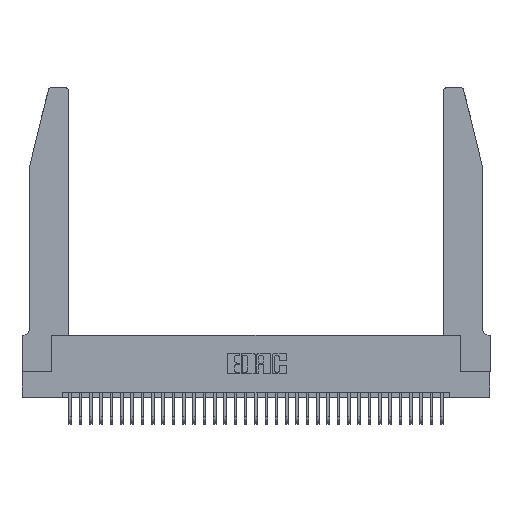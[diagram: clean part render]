
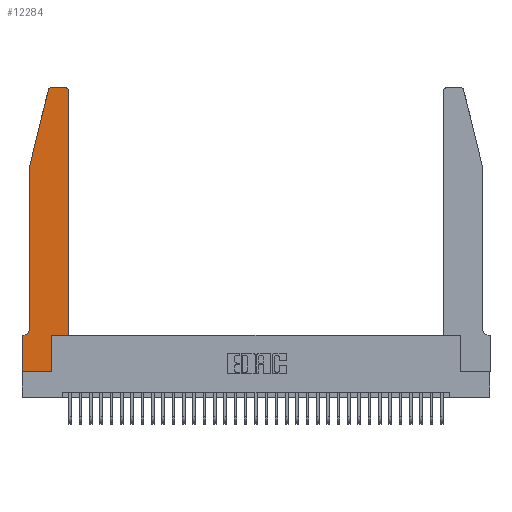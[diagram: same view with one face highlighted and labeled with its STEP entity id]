
A CAD part, top view. The second image highlights one B-rep face of the part: STEP entity #12284.
In plain terms, the highlighted planar face has unit normal (0, 0, 1).
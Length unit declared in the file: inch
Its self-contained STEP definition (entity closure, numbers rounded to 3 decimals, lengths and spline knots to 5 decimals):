
#522 = EDGE_CURVE ( 'NONE', #15158, #9549, #29890, .T. ) ;
#568 = LINE ( 'NONE', #18574, #27272 ) ;
#1459 = DIRECTION ( 'NONE',  ( -1., 0., 0. ) ) ;
#1544 = DIRECTION ( 'NONE',  ( 0., 0., 1. ) ) ;
#1998 = FACE_OUTER_BOUND ( 'NONE', #5736, .T. ) ;
#2839 = CARTESIAN_POINT ( 'NONE',  ( 0.0755, 2., 0.37 ) ) ;
#2873 = CARTESIAN_POINT ( 'NONE',  ( 0.2865, 0., 0.37 ) ) ;
#3316 = CARTESIAN_POINT ( 'NONE',  ( 0.4205, 2.75, 0.37 ) ) ;
#3374 = EDGE_CURVE ( 'NONE', #4253, #15158, #20533, .T. ) ;
#4253 = VERTEX_POINT ( 'NONE', #31362 ) ;
#4255 = EDGE_CURVE ( 'NONE', #18938, #19141, #568, .T. ) ;
#4879 = VERTEX_POINT ( 'NONE', #28804 ) ;
#4895 = DIRECTION ( 'NONE',  ( 0., 0., 1. ) ) ;
#5441 = CARTESIAN_POINT ( 'NONE',  ( 0.4505, 0.35, 0.37 ) ) ;
#5593 = EDGE_CURVE ( 'NONE', #32367, #4879, #26120, .T. ) ;
#5736 = EDGE_LOOP ( 'NONE', ( #17999, #22004, #30364, #19204, #9488, #18029, #5848, #23654, #18455, #13189, #17225, #11971 ) ) ;
#5848 = ORIENTED_EDGE ( 'NONE', *, *, #13122, .T. ) ;
#5872 = DIRECTION ( 'NONE',  ( 0., 0., -1. ) ) ;
#7199 = CARTESIAN_POINT ( 'NONE',  ( 0.0755, 0.42, 0.37 ) ) ;
#7503 = EDGE_CURVE ( 'NONE', #4879, #18938, #32324, .T. ) ;
#7509 = AXIS2_PLACEMENT_3D ( 'NONE', #8967, #26994, #11577 ) ;
#8612 = VECTOR ( 'NONE', #14992, 39.37008 ) ;
#8967 = CARTESIAN_POINT ( 'NONE',  ( 0.284, 2.72, 0.37 ) ) ;
#9488 = ORIENTED_EDGE ( 'NONE', *, *, #32392, .T. ) ;
#9549 = VERTEX_POINT ( 'NONE', #17577 ) ;
#9755 = CARTESIAN_POINT ( 'NONE',  ( 0., 0., 0.37 ) ) ;
#10136 = EDGE_CURVE ( 'NONE', #9549, #29357, #19407, .T. ) ;
#10212 = CARTESIAN_POINT ( 'NONE',  ( 0.2605, 2.75, 0.37 ) ) ;
#10248 = LINE ( 'NONE', #17865, #22350 ) ;
#11153 = LINE ( 'NONE', #19621, #17193 ) ;
#11577 = DIRECTION ( 'NONE',  ( 1., 0., 0. ) ) ;
#11908 = VECTOR ( 'NONE', #29328, 39.37008 ) ;
#11971 = ORIENTED_EDGE ( 'NONE', *, *, #10136, .T. ) ;
#12284 = ADVANCED_FACE ( 'NONE', ( #1998 ), #32400, .T. ) ;
#13122 = EDGE_CURVE ( 'NONE', #14083, #20221, #17404, .T. ) ;
#13189 = ORIENTED_EDGE ( 'NONE', *, *, #3374, .T. ) ;
#13206 = EDGE_CURVE ( 'NONE', #29357, #32367, #13377, .T. ) ;
#13377 = LINE ( 'NONE', #10212, #26264 ) ;
#14083 = VERTEX_POINT ( 'NONE', #29036 ) ;
#14992 = DIRECTION ( 'NONE',  ( 1., 0., 0. ) ) ;
#15158 = VERTEX_POINT ( 'NONE', #27956 ) ;
#15182 = DIRECTION ( 'NONE',  ( 0., 1., 0. ) ) ;
#15446 = DIRECTION ( 'NONE',  ( -1., 0., 0. ) ) ;
#15706 = VERTEX_POINT ( 'NONE', #23068 ) ;
#17193 = VECTOR ( 'NONE', #1459, 39.37008 ) ;
#17225 = ORIENTED_EDGE ( 'NONE', *, *, #522, .T. ) ;
#17404 = LINE ( 'NONE', #32818, #23449 ) ;
#17577 = CARTESIAN_POINT ( 'NONE',  ( 0.4505, 2.72, 0.37 ) ) ;
#17865 = CARTESIAN_POINT ( 'NONE',  ( 0.2865, 0.35, 0.37 ) ) ;
#17999 = ORIENTED_EDGE ( 'NONE', *, *, #13206, .T. ) ;
#18029 = ORIENTED_EDGE ( 'NONE', *, *, #19073, .T. ) ;
#18455 = ORIENTED_EDGE ( 'NONE', *, *, #32812, .T. ) ;
#18574 = CARTESIAN_POINT ( 'NONE',  ( 0.0755, 2., 0.37 ) ) ;
#18680 = DIRECTION ( 'NONE',  ( 0., -1., 0. ) ) ;
#18938 = VERTEX_POINT ( 'NONE', #2839 ) ;
#19073 = EDGE_CURVE ( 'NONE', #15706, #14083, #11153, .T. ) ;
#19141 = VERTEX_POINT ( 'NONE', #7199 ) ;
#19204 = ORIENTED_EDGE ( 'NONE', *, *, #4255, .T. ) ;
#19407 = CIRCLE ( 'NONE', #25103, 0.03 ) ;
#19621 = CARTESIAN_POINT ( 'NONE',  ( 0.0755, 0.35, 0.37 ) ) ;
#19713 = DIRECTION ( 'NONE',  ( 1., 0., 0. ) ) ;
#20221 = VERTEX_POINT ( 'NONE', #29180 ) ;
#20427 = CARTESIAN_POINT ( 'NONE',  ( 0.4205, 2.72, 0.37 ) ) ;
#20432 = DIRECTION ( 'NONE',  ( 0., 1., 0. ) ) ;
#20533 = LINE ( 'NONE', #5441, #32455 ) ;
#21373 = CARTESIAN_POINT ( 'NONE',  ( 0.0055, 0.42, 0.37 ) ) ;
#22004 = ORIENTED_EDGE ( 'NONE', *, *, #5593, .T. ) ;
#22350 = VECTOR ( 'NONE', #20432, 39.37008 ) ;
#22750 = DIRECTION ( 'NONE',  ( 0., -1., 0. ) ) ;
#22777 = CARTESIAN_POINT ( 'NONE',  ( 0.4505, 0.35, 0.37 ) ) ;
#23037 = DIRECTION ( 'NONE',  ( 1., 0., 0. ) ) ;
#23068 = CARTESIAN_POINT ( 'NONE',  ( 0.0055, 0.35, 0.37 ) ) ;
#23155 = VECTOR ( 'NONE', #15182, 39.37008 ) ;
#23449 = VECTOR ( 'NONE', #22750, 39.37008 ) ;
#23654 = ORIENTED_EDGE ( 'NONE', *, *, #25053, .T. ) ;
#23852 = CARTESIAN_POINT ( 'NONE',  ( 0.284, 2.75, 0.37 ) ) ;
#23957 = DIRECTION ( 'NONE',  ( -1., 0., 0. ) ) ;
#24233 = CARTESIAN_POINT ( 'NONE',  ( 0.0755, 2., 0.37 ) ) ;
#24795 = CARTESIAN_POINT ( 'NONE',  ( 0., 0.35, 0.37 ) ) ;
#25053 = EDGE_CURVE ( 'NONE', #20221, #32319, #29130, .T. ) ;
#25103 = AXIS2_PLACEMENT_3D ( 'NONE', #20427, #4895, #23037 ) ;
#26120 = CIRCLE ( 'NONE', #7509, 0.03 ) ;
#26264 = VECTOR ( 'NONE', #15446, 39.37008 ) ;
#26994 = DIRECTION ( 'NONE',  ( 0., 0., 1. ) ) ;
#27272 = VECTOR ( 'NONE', #18680, 39.37008 ) ;
#27426 = AXIS2_PLACEMENT_3D ( 'NONE', #21373, #5872, #23957 ) ;
#27956 = CARTESIAN_POINT ( 'NONE',  ( 0.4505, 0.35, 0.37 ) ) ;
#28804 = CARTESIAN_POINT ( 'NONE',  ( 0.25487, 2.72718, 0.37 ) ) ;
#29036 = CARTESIAN_POINT ( 'NONE',  ( 0., 0.35, 0.37 ) ) ;
#29130 = LINE ( 'NONE', #9755, #8612 ) ;
#29180 = CARTESIAN_POINT ( 'NONE',  ( 0., 0., 0.37 ) ) ;
#29328 = DIRECTION ( 'NONE',  ( -0.239, -0.971, 0. ) ) ;
#29357 = VERTEX_POINT ( 'NONE', #3316 ) ;
#29495 = CIRCLE ( 'NONE', #27426, 0.07 ) ;
#29890 = LINE ( 'NONE', #22777, #23155 ) ;
#30364 = ORIENTED_EDGE ( 'NONE', *, *, #7503, .T. ) ;
#31176 = DIRECTION ( 'NONE',  ( 1., 0., 0. ) ) ;
#31362 = CARTESIAN_POINT ( 'NONE',  ( 0.2865, 0.35, 0.37 ) ) ;
#32319 = VERTEX_POINT ( 'NONE', #2873 ) ;
#32324 = LINE ( 'NONE', #24233, #11908 ) ;
#32367 = VERTEX_POINT ( 'NONE', #23852 ) ;
#32392 = EDGE_CURVE ( 'NONE', #19141, #15706, #29495, .T. ) ;
#32400 = PLANE ( 'NONE',  #33274 ) ;
#32455 = VECTOR ( 'NONE', #31176, 39.37008 ) ;
#32812 = EDGE_CURVE ( 'NONE', #32319, #4253, #10248, .T. ) ;
#32818 = CARTESIAN_POINT ( 'NONE',  ( 0., 0., 0.37 ) ) ;
#33274 = AXIS2_PLACEMENT_3D ( 'NONE', #24795, #1544, #19713 ) ;
